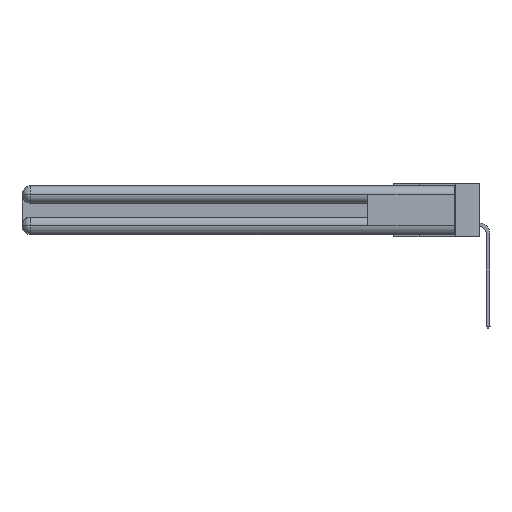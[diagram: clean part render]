
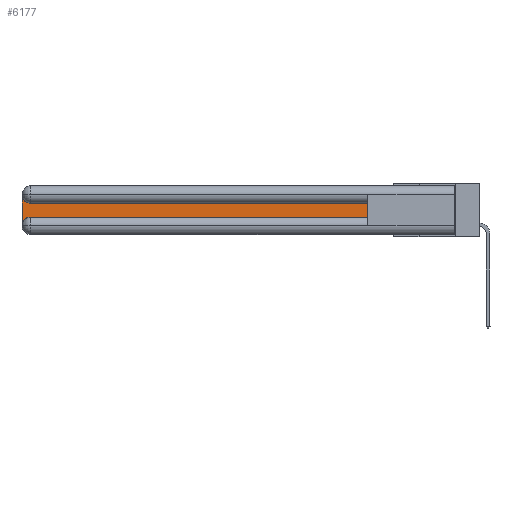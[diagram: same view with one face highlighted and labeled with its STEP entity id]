
A CAD part, left-side view. The second image highlights one B-rep face of the part: STEP entity #6177.
In plain terms, the highlighted planar face has unit normal (-1, 0, 0).
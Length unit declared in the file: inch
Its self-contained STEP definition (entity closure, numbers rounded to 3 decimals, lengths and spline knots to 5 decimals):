
#152 = CARTESIAN_POINT ( 'NONE',  ( 0.075, 2.94, -0.2775 ) ) ;
#1480 = AXIS2_PLACEMENT_3D ( 'NONE', #20290, #31020, #12808 ) ;
#1834 = EDGE_CURVE ( 'NONE', #34007, #33869, #10594, .T. ) ;
#2917 = VERTEX_POINT ( 'NONE', #5378 ) ;
#3902 = ORIENTED_EDGE ( 'NONE', *, *, #29349, .T. ) ;
#4465 = CIRCLE ( 'NONE', #6800, 0.06 ) ;
#4599 = CARTESIAN_POINT ( 'NONE',  ( 0.075, 3., -0.2775 ) ) ;
#4994 = VERTEX_POINT ( 'NONE', #22678 ) ;
#5378 = CARTESIAN_POINT ( 'NONE',  ( 0.075, 0.6, -0.1225 ) ) ;
#6177 = ADVANCED_FACE ( 'NONE', ( #31350 ), #33594, .F. ) ;
#6800 = AXIS2_PLACEMENT_3D ( 'NONE', #152, #10507, #18473 ) ;
#8109 = ORIENTED_EDGE ( 'NONE', *, *, #1834, .T. ) ;
#9236 = EDGE_CURVE ( 'NONE', #4994, #34007, #20313, .T. ) ;
#9460 = VECTOR ( 'NONE', #29655, 39.37008 ) ;
#9744 = DIRECTION ( 'NONE',  ( 0., -1., 0. ) ) ;
#9772 = VECTOR ( 'NONE', #22584, 39.37008 ) ;
#9891 = ORIENTED_EDGE ( 'NONE', *, *, #12441, .T. ) ;
#10507 = DIRECTION ( 'NONE',  ( 1., 0., 0. ) ) ;
#10594 = LINE ( 'NONE', #32900, #9772 ) ;
#10903 = VERTEX_POINT ( 'NONE', #30380 ) ;
#11341 = DIRECTION ( 'NONE',  ( 0., 1., 0. ) ) ;
#11467 = ORIENTED_EDGE ( 'NONE', *, *, #9236, .T. ) ;
#12201 = DIRECTION ( 'NONE',  ( 0., 0., -1. ) ) ;
#12441 = EDGE_CURVE ( 'NONE', #21403, #2917, #16457, .T. ) ;
#12808 = DIRECTION ( 'NONE',  ( 0., 0., -1. ) ) ;
#13059 = LINE ( 'NONE', #32104, #17582 ) ;
#13131 = EDGE_CURVE ( 'NONE', #33869, #10903, #4465, .T. ) ;
#14943 = CARTESIAN_POINT ( 'NONE',  ( 0.075, 2.94, -0.0625 ) ) ;
#15639 = LINE ( 'NONE', #30640, #21820 ) ;
#16457 = LINE ( 'NONE', #24977, #9460 ) ;
#17582 = VECTOR ( 'NONE', #11341, 39.37008 ) ;
#18473 = DIRECTION ( 'NONE',  ( 0., 0., -1. ) ) ;
#19182 = ORIENTED_EDGE ( 'NONE', *, *, #13131, .T. ) ;
#20290 = CARTESIAN_POINT ( 'NONE',  ( 0.075, 3., -0.1225 ) ) ;
#20313 = CIRCLE ( 'NONE', #31884, 0.06 ) ;
#21403 = VERTEX_POINT ( 'NONE', #32055 ) ;
#21820 = VECTOR ( 'NONE', #9744, 39.37008 ) ;
#22584 = DIRECTION ( 'NONE',  ( 0., 0., -1. ) ) ;
#22678 = CARTESIAN_POINT ( 'NONE',  ( 0.075, 2.94, -0.1225 ) ) ;
#22818 = EDGE_LOOP ( 'NONE', ( #23690, #11467, #8109, #19182, #3902, #9891 ) ) ;
#22983 = DIRECTION ( 'NONE',  ( 1., 0., 0. ) ) ;
#23560 = CARTESIAN_POINT ( 'NONE',  ( 0.075, 3., -0.0625 ) ) ;
#23690 = ORIENTED_EDGE ( 'NONE', *, *, #30590, .T. ) ;
#24977 = CARTESIAN_POINT ( 'NONE',  ( 0.075, 0.6, -0.2175 ) ) ;
#29349 = EDGE_CURVE ( 'NONE', #10903, #21403, #15639, .T. ) ;
#29655 = DIRECTION ( 'NONE',  ( 0., 0., 1. ) ) ;
#30380 = CARTESIAN_POINT ( 'NONE',  ( 0.075, 2.94, -0.2175 ) ) ;
#30590 = EDGE_CURVE ( 'NONE', #2917, #4994, #13059, .T. ) ;
#30640 = CARTESIAN_POINT ( 'NONE',  ( 0.075, 0.6, -0.2175 ) ) ;
#31020 = DIRECTION ( 'NONE',  ( 1., 0., 0. ) ) ;
#31350 = FACE_OUTER_BOUND ( 'NONE', #22818, .T. ) ;
#31884 = AXIS2_PLACEMENT_3D ( 'NONE', #14943, #22983, #12201 ) ;
#32055 = CARTESIAN_POINT ( 'NONE',  ( 0.075, 0.6, -0.2175 ) ) ;
#32104 = CARTESIAN_POINT ( 'NONE',  ( 0.075, 0.6, -0.1225 ) ) ;
#32900 = CARTESIAN_POINT ( 'NONE',  ( 0.075, 3., -0.2175 ) ) ;
#33594 = PLANE ( 'NONE',  #1480 ) ;
#33869 = VERTEX_POINT ( 'NONE', #4599 ) ;
#34007 = VERTEX_POINT ( 'NONE', #23560 ) ;
